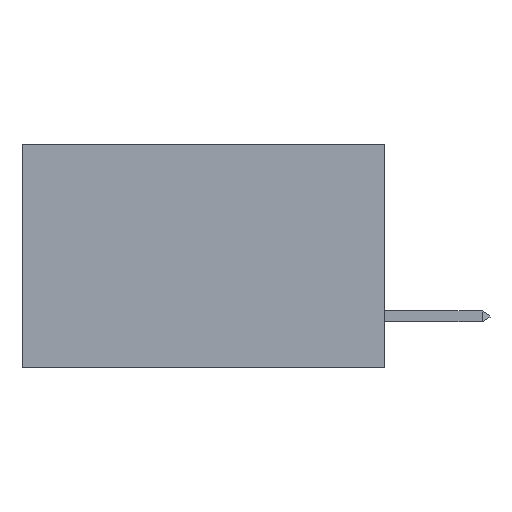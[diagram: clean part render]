
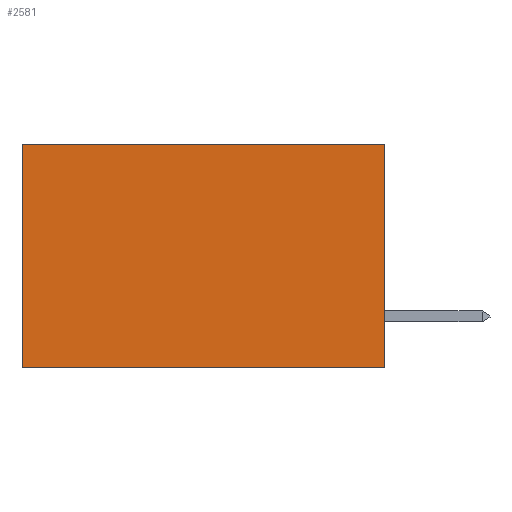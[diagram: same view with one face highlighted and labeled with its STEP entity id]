
A CAD part, left-side view. The second image highlights one B-rep face of the part: STEP entity #2581.
In plain terms, the highlighted planar face has unit normal (-1, 0, 0).
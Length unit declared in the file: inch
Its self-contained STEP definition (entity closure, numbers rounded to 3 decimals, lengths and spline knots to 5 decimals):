
#390 = DIRECTION ( 'NONE',  ( 0., 0., -1. ) ) ;
#444 = DIRECTION ( 'NONE',  ( 0., 0., -1. ) ) ;
#754 = VERTEX_POINT ( 'NONE', #8235 ) ;
#1118 = LINE ( 'NONE', #8554, #4815 ) ;
#1326 = DIRECTION ( 'NONE',  ( 0., 0., -1. ) ) ;
#1680 = DIRECTION ( 'NONE',  ( 1., 0., 0. ) ) ;
#1787 = CARTESIAN_POINT ( 'NONE',  ( 0.2875, 0.6, 0. ) ) ;
#2174 = ORIENTED_EDGE ( 'NONE', *, *, #3730, .T. ) ;
#2190 = ORIENTED_EDGE ( 'NONE', *, *, #8815, .F. ) ;
#2581 = ADVANCED_FACE ( 'NONE', ( #10160 ), #7039, .F. ) ;
#2582 = VECTOR ( 'NONE', #390, 39.37008 ) ;
#3730 = EDGE_CURVE ( 'NONE', #3860, #7714, #10135, .T. ) ;
#3774 = CARTESIAN_POINT ( 'NONE',  ( 0.2875, 0.6, 0. ) ) ;
#3860 = VERTEX_POINT ( 'NONE', #3774 ) ;
#4468 = VECTOR ( 'NONE', #444, 39.37008 ) ;
#4484 = ORIENTED_EDGE ( 'NONE', *, *, #8718, .T. ) ;
#4815 = VECTOR ( 'NONE', #9209, 39.37008 ) ;
#4837 = LINE ( 'NONE', #9369, #2582 ) ;
#5261 = VECTOR ( 'NONE', #9961, 39.37008 ) ;
#5282 = EDGE_CURVE ( 'NONE', #7386, #7714, #1118, .T. ) ;
#6354 = CARTESIAN_POINT ( 'NONE',  ( 0.2875, 0., 0. ) ) ;
#6824 = CARTESIAN_POINT ( 'NONE',  ( 0.2875, 0.6, -0.37 ) ) ;
#7039 = PLANE ( 'NONE',  #9756 ) ;
#7296 = EDGE_LOOP ( 'NONE', ( #2174, #10375, #2190, #4484 ) ) ;
#7380 = LINE ( 'NONE', #9270, #5261 ) ;
#7386 = VERTEX_POINT ( 'NONE', #7980 ) ;
#7714 = VERTEX_POINT ( 'NONE', #6824 ) ;
#7980 = CARTESIAN_POINT ( 'NONE',  ( 0.2875, 0., -0.37 ) ) ;
#8235 = CARTESIAN_POINT ( 'NONE',  ( 0.2875, 0., 0. ) ) ;
#8554 = CARTESIAN_POINT ( 'NONE',  ( 0.2875, 0., -0.37 ) ) ;
#8718 = EDGE_CURVE ( 'NONE', #754, #3860, #7380, .T. ) ;
#8815 = EDGE_CURVE ( 'NONE', #754, #7386, #4837, .T. ) ;
#9209 = DIRECTION ( 'NONE',  ( 0., 1., 0. ) ) ;
#9270 = CARTESIAN_POINT ( 'NONE',  ( 0.2875, 0., 0. ) ) ;
#9369 = CARTESIAN_POINT ( 'NONE',  ( 0.2875, 0., 0. ) ) ;
#9756 = AXIS2_PLACEMENT_3D ( 'NONE', #6354, #1680, #1326 ) ;
#9961 = DIRECTION ( 'NONE',  ( 0., 1., 0. ) ) ;
#10135 = LINE ( 'NONE', #1787, #4468 ) ;
#10160 = FACE_OUTER_BOUND ( 'NONE', #7296, .T. ) ;
#10375 = ORIENTED_EDGE ( 'NONE', *, *, #5282, .F. ) ;
